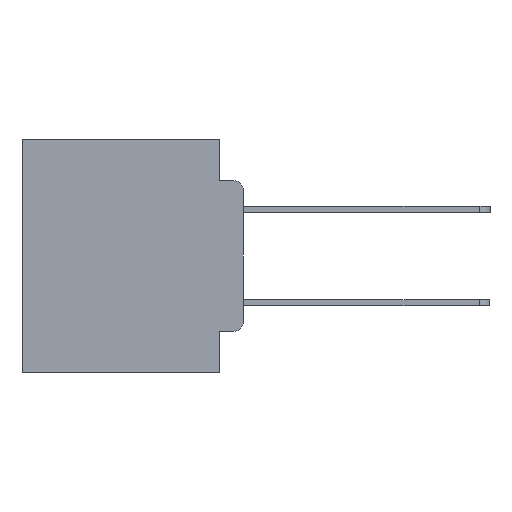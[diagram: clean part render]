
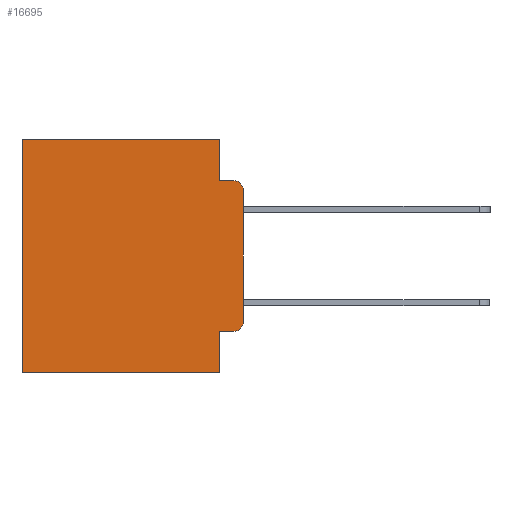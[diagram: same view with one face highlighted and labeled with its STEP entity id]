
A CAD part, left-side view. The second image highlights one B-rep face of the part: STEP entity #16695.
In plain terms, the highlighted planar face has unit normal (-1, 0, 0).
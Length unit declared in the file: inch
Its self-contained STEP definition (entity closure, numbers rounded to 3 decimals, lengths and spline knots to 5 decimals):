
#522 = VERTEX_POINT ( 'NONE', #17681 ) ;
#957 = CARTESIAN_POINT ( 'NONE',  ( 0.298, 0.051, 0. ) ) ;
#1063 = EDGE_CURVE ( 'NONE', #9736, #8459, #14555, .T. ) ;
#1185 = EDGE_LOOP ( 'NONE', ( #9811, #4310, #11105, #19635, #10432, #15758, #7948, #3101, #6122, #22510 ) ) ;
#1723 = LINE ( 'NONE', #17746, #8559 ) ;
#1919 = DIRECTION ( 'NONE',  ( 0., 0., -1. ) ) ;
#3100 = DIRECTION ( 'NONE',  ( 0., 0., -1. ) ) ;
#3101 = ORIENTED_EDGE ( 'NONE', *, *, #17029, .F. ) ;
#3525 = DIRECTION ( 'NONE',  ( -1., 0., 0. ) ) ;
#3928 = EDGE_CURVE ( 'NONE', #14620, #14851, #25219, .T. ) ;
#4061 = DIRECTION ( 'NONE',  ( 0., 0., -1. ) ) ;
#4310 = ORIENTED_EDGE ( 'NONE', *, *, #3928, .T. ) ;
#4754 = EDGE_CURVE ( 'NONE', #8665, #9736, #8995, .T. ) ;
#5127 = EDGE_CURVE ( 'NONE', #13110, #15989, #15024, .T. ) ;
#5236 = VERTEX_POINT ( 'NONE', #14123 ) ;
#5451 = AXIS2_PLACEMENT_3D ( 'NONE', #16930, #24049, #21948 ) ;
#5698 = DIRECTION ( 'NONE',  ( 0., 0., -1. ) ) ;
#5755 = EDGE_CURVE ( 'NONE', #14620, #15989, #1723, .T. ) ;
#5827 = DIRECTION ( 'NONE',  ( 0., -1., 0. ) ) ;
#6122 = ORIENTED_EDGE ( 'NONE', *, *, #12684, .T. ) ;
#6160 = AXIS2_PLACEMENT_3D ( 'NONE', #15751, #3525, #17694 ) ;
#6473 = EDGE_CURVE ( 'NONE', #12018, #8459, #6937, .T. ) ;
#6478 = DIRECTION ( 'NONE',  ( 0., 1., 0. ) ) ;
#6937 = LINE ( 'NONE', #23532, #11721 ) ;
#7080 = LINE ( 'NONE', #957, #17125 ) ;
#7562 = CARTESIAN_POINT ( 'NONE',  ( 0.298, 0.051, -0.5 ) ) ;
#7882 = CARTESIAN_POINT ( 'NONE',  ( 0.298, 0.051, -0.4115 ) ) ;
#7927 = VECTOR ( 'NONE', #17339, 39.37008 ) ;
#7948 = ORIENTED_EDGE ( 'NONE', *, *, #6473, .F. ) ;
#7975 = CARTESIAN_POINT ( 'NONE',  ( 0.298, 0.02, -0.0885 ) ) ;
#8073 = LINE ( 'NONE', #14265, #18099 ) ;
#8102 = PLANE ( 'NONE',  #9104 ) ;
#8459 = VERTEX_POINT ( 'NONE', #10817 ) ;
#8559 = VECTOR ( 'NONE', #5698, 39.37008 ) ;
#8665 = VERTEX_POINT ( 'NONE', #21326 ) ;
#8995 = LINE ( 'NONE', #18489, #13783 ) ;
#9104 = AXIS2_PLACEMENT_3D ( 'NONE', #25759, #14269, #1919 ) ;
#9144 = VECTOR ( 'NONE', #22048, 39.37008 ) ;
#9214 = LINE ( 'NONE', #13410, #7927 ) ;
#9736 = VERTEX_POINT ( 'NONE', #22535 ) ;
#9811 = ORIENTED_EDGE ( 'NONE', *, *, #5755, .F. ) ;
#10432 = ORIENTED_EDGE ( 'NONE', *, *, #4754, .T. ) ;
#10817 = CARTESIAN_POINT ( 'NONE',  ( 0.298, 0.473, -0.5 ) ) ;
#11105 = ORIENTED_EDGE ( 'NONE', *, *, #23503, .F. ) ;
#11721 = VECTOR ( 'NONE', #13887, 39.37008 ) ;
#12018 = VERTEX_POINT ( 'NONE', #7562 ) ;
#12684 = EDGE_CURVE ( 'NONE', #5236, #13110, #18547, .T. ) ;
#13110 = VERTEX_POINT ( 'NONE', #22213 ) ;
#13410 = CARTESIAN_POINT ( 'NONE',  ( 0.298, 0.051, -0.0885 ) ) ;
#13783 = VECTOR ( 'NONE', #6478, 39.37008 ) ;
#13887 = DIRECTION ( 'NONE',  ( 0., 1., 0. ) ) ;
#14123 = CARTESIAN_POINT ( 'NONE',  ( 0.298, 0.051, -0.4115 ) ) ;
#14265 = CARTESIAN_POINT ( 'NONE',  ( 0.298, 0.051, 0. ) ) ;
#14269 = DIRECTION ( 'NONE',  ( 1., 0., 0. ) ) ;
#14555 = LINE ( 'NONE', #18990, #9144 ) ;
#14620 = VERTEX_POINT ( 'NONE', #17380 ) ;
#14851 = VERTEX_POINT ( 'NONE', #7975 ) ;
#15024 = CIRCLE ( 'NONE', #6160, 0.02 ) ;
#15751 = CARTESIAN_POINT ( 'NONE',  ( 0.298, 0.02, -0.3915 ) ) ;
#15758 = ORIENTED_EDGE ( 'NONE', *, *, #1063, .T. ) ;
#15989 = VERTEX_POINT ( 'NONE', #19762 ) ;
#16695 = ADVANCED_FACE ( 'NONE', ( #24365 ), #8102, .F. ) ;
#16930 = CARTESIAN_POINT ( 'NONE',  ( 0.298, 0.02, -0.1085 ) ) ;
#17029 = EDGE_CURVE ( 'NONE', #5236, #12018, #7080, .T. ) ;
#17125 = VECTOR ( 'NONE', #3100, 39.37008 ) ;
#17339 = DIRECTION ( 'NONE',  ( 0., -1., 0. ) ) ;
#17380 = CARTESIAN_POINT ( 'NONE',  ( 0.298, 0., -0.1085 ) ) ;
#17681 = CARTESIAN_POINT ( 'NONE',  ( 0.298, 0.051, -0.0885 ) ) ;
#17694 = DIRECTION ( 'NONE',  ( 0., 0., -1. ) ) ;
#17746 = CARTESIAN_POINT ( 'NONE',  ( 0.298, 0., 0. ) ) ;
#18099 = VECTOR ( 'NONE', #4061, 39.37008 ) ;
#18489 = CARTESIAN_POINT ( 'NONE',  ( 0.298, 0., 0. ) ) ;
#18547 = LINE ( 'NONE', #7882, #23067 ) ;
#18990 = CARTESIAN_POINT ( 'NONE',  ( 0.298, 0.473, 0. ) ) ;
#19635 = ORIENTED_EDGE ( 'NONE', *, *, #20946, .F. ) ;
#19762 = CARTESIAN_POINT ( 'NONE',  ( 0.298, 0., -0.3915 ) ) ;
#20946 = EDGE_CURVE ( 'NONE', #8665, #522, #8073, .T. ) ;
#21326 = CARTESIAN_POINT ( 'NONE',  ( 0.298, 0.051, 0. ) ) ;
#21948 = DIRECTION ( 'NONE',  ( 0., 0., -1. ) ) ;
#22048 = DIRECTION ( 'NONE',  ( 0., 0., -1. ) ) ;
#22213 = CARTESIAN_POINT ( 'NONE',  ( 0.298, 0.02, -0.4115 ) ) ;
#22510 = ORIENTED_EDGE ( 'NONE', *, *, #5127, .T. ) ;
#22535 = CARTESIAN_POINT ( 'NONE',  ( 0.298, 0.473, 0. ) ) ;
#23067 = VECTOR ( 'NONE', #5827, 39.37008 ) ;
#23503 = EDGE_CURVE ( 'NONE', #522, #14851, #9214, .T. ) ;
#23532 = CARTESIAN_POINT ( 'NONE',  ( 0.298, 0., -0.5 ) ) ;
#24049 = DIRECTION ( 'NONE',  ( -1., 0., 0. ) ) ;
#24365 = FACE_OUTER_BOUND ( 'NONE', #1185, .T. ) ;
#25219 = CIRCLE ( 'NONE', #5451, 0.02 ) ;
#25759 = CARTESIAN_POINT ( 'NONE',  ( 0.298, 0., 0. ) ) ;
